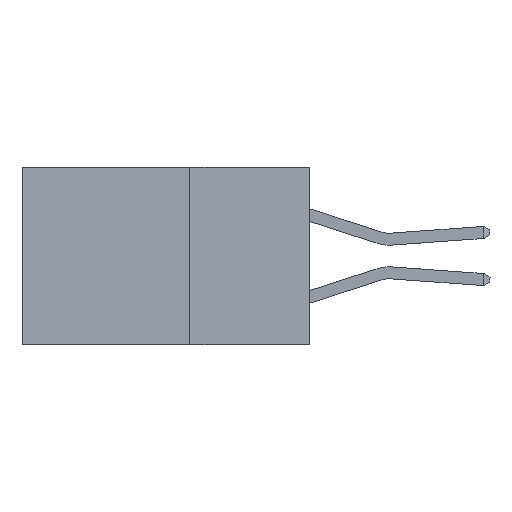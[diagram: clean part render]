
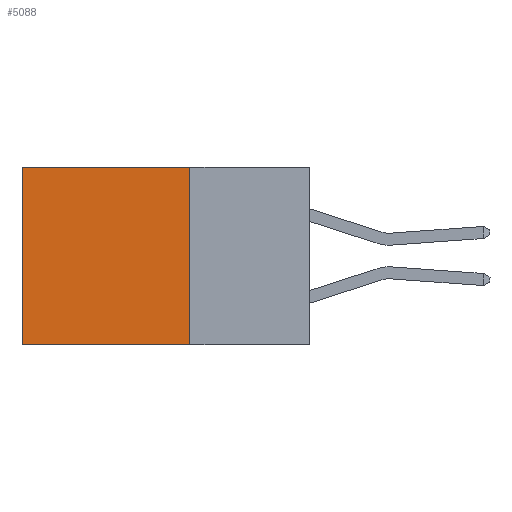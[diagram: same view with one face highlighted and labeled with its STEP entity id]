
A CAD part, left-side view. The second image highlights one B-rep face of the part: STEP entity #5088.
In plain terms, the highlighted planar face has unit normal (-1, 0, 0).
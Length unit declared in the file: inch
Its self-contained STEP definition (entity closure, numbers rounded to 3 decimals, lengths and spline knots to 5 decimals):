
#191 = VERTEX_POINT ( 'NONE', #8051 ) ;
#492 = EDGE_LOOP ( 'NONE', ( #5523, #3060, #6046, #4721 ) ) ;
#1194 = CARTESIAN_POINT ( 'NONE',  ( 0.298, 0.25, 0. ) ) ;
#2030 = VECTOR ( 'NONE', #6782, 39.37008 ) ;
#2422 = LINE ( 'NONE', #10419, #2030 ) ;
#2752 = DIRECTION ( 'NONE',  ( 0., 0., -1. ) ) ;
#3060 = ORIENTED_EDGE ( 'NONE', *, *, #9492, .F. ) ;
#3350 = VERTEX_POINT ( 'NONE', #4577 ) ;
#3544 = CARTESIAN_POINT ( 'NONE',  ( 0.298, 0.25, -0.37 ) ) ;
#3798 = AXIS2_PLACEMENT_3D ( 'NONE', #11255, #11401, #2752 ) ;
#3875 = LINE ( 'NONE', #7265, #9024 ) ;
#4577 = CARTESIAN_POINT ( 'NONE',  ( 0.298, 0.6, -0.37 ) ) ;
#4721 = ORIENTED_EDGE ( 'NONE', *, *, #11047, .T. ) ;
#5088 = ADVANCED_FACE ( 'NONE', ( #10121 ), #7506, .F. ) ;
#5523 = ORIENTED_EDGE ( 'NONE', *, *, #11433, .T. ) ;
#5529 = CARTESIAN_POINT ( 'NONE',  ( 0.298, 0.6, 0. ) ) ;
#6046 = ORIENTED_EDGE ( 'NONE', *, *, #9402, .F. ) ;
#6782 = DIRECTION ( 'NONE',  ( 0., 0., -1. ) ) ;
#7265 = CARTESIAN_POINT ( 'NONE',  ( 0.298, 0.25, 0. ) ) ;
#7506 = PLANE ( 'NONE',  #3798 ) ;
#7758 = VERTEX_POINT ( 'NONE', #15426 ) ;
#7939 = LINE ( 'NONE', #3544, #14868 ) ;
#8051 = CARTESIAN_POINT ( 'NONE',  ( 0.298, 0.6, 0. ) ) ;
#9024 = VECTOR ( 'NONE', #14415, 39.37008 ) ;
#9402 = EDGE_CURVE ( 'NONE', #12516, #7758, #2422, .T. ) ;
#9492 = EDGE_CURVE ( 'NONE', #7758, #3350, #7939, .T. ) ;
#10121 = FACE_OUTER_BOUND ( 'NONE', #492, .T. ) ;
#10328 = DIRECTION ( 'NONE',  ( 0., 0., -1. ) ) ;
#10419 = CARTESIAN_POINT ( 'NONE',  ( 0.298, 0.25, 0. ) ) ;
#11047 = EDGE_CURVE ( 'NONE', #12516, #191, #3875, .T. ) ;
#11255 = CARTESIAN_POINT ( 'NONE',  ( 0.298, 0.25, 0. ) ) ;
#11401 = DIRECTION ( 'NONE',  ( 1., 0., 0. ) ) ;
#11433 = EDGE_CURVE ( 'NONE', #191, #3350, #15193, .T. ) ;
#12516 = VERTEX_POINT ( 'NONE', #1194 ) ;
#13595 = DIRECTION ( 'NONE',  ( 0., 1., 0. ) ) ;
#14415 = DIRECTION ( 'NONE',  ( 0., 1., 0. ) ) ;
#14598 = VECTOR ( 'NONE', #10328, 39.37008 ) ;
#14868 = VECTOR ( 'NONE', #13595, 39.37008 ) ;
#15193 = LINE ( 'NONE', #5529, #14598 ) ;
#15426 = CARTESIAN_POINT ( 'NONE',  ( 0.298, 0.25, -0.37 ) ) ;
